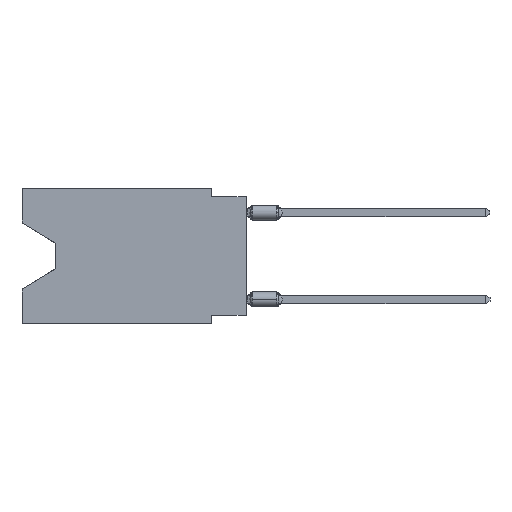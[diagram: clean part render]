
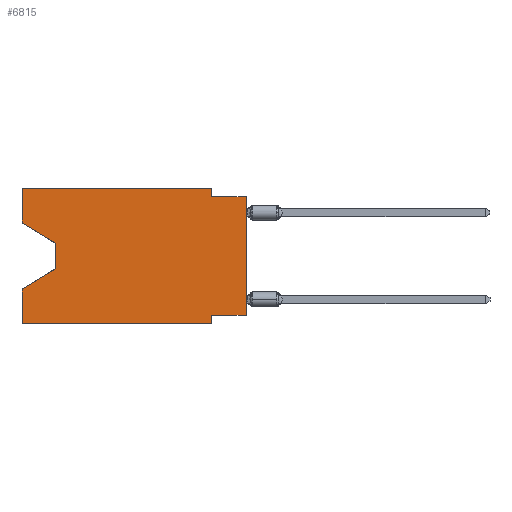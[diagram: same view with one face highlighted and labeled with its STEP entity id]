
A CAD part, left-side view. The second image highlights one B-rep face of the part: STEP entity #6815.
In plain terms, the highlighted planar face has unit normal (-1, 0, 0).
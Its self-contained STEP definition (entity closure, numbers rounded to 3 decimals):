
#292 = DIRECTION ( 'NONE',  ( 1., 0., 0. ) ) ;
#353 = VERTEX_POINT ( 'NONE', #10579 ) ;
#389 = EDGE_CURVE ( 'NONE', #13629, #1016, #3475, .T. ) ;
#968 = VECTOR ( 'NONE', #1400, 1000. ) ;
#1016 = VERTEX_POINT ( 'NONE', #14931 ) ;
#1067 = EDGE_CURVE ( 'NONE', #29259, #17591, #10344, .T. ) ;
#1400 = DIRECTION ( 'NONE',  ( 0., 0., 1. ) ) ;
#2330 = CARTESIAN_POINT ( 'NONE',  ( 0., 16.383, -9.906 ) ) ;
#2386 = CARTESIAN_POINT ( 'NONE',  ( 0., 0., -9.271 ) ) ;
#2411 = CARTESIAN_POINT ( 'NONE',  ( 0., 2.54, -9.906 ) ) ;
#3475 = LINE ( 'NONE', #3944, #26967 ) ;
#3944 = CARTESIAN_POINT ( 'NONE',  ( 0., 13.97, -4.013 ) ) ;
#4146 = VERTEX_POINT ( 'NONE', #13972 ) ;
#5473 = VECTOR ( 'NONE', #10708, 1000. ) ;
#5491 = LINE ( 'NONE', #27127, #30557 ) ;
#5962 = VECTOR ( 'NONE', #19684, 1000. ) ;
#6553 = DIRECTION ( 'NONE',  ( 0., -1., 0. ) ) ;
#6568 = CARTESIAN_POINT ( 'NONE',  ( 0., 0., -0.635 ) ) ;
#6754 = CARTESIAN_POINT ( 'NONE',  ( 0., 16.383, 0. ) ) ;
#6815 = ADVANCED_FACE ( 'NONE', ( #24852 ), #7393, .F. ) ;
#7220 = DIRECTION ( 'NONE',  ( 0., -1., 0. ) ) ;
#7393 = PLANE ( 'NONE',  #9376 ) ;
#7778 = CARTESIAN_POINT ( 'NONE',  ( 0., 16.383, -2.546 ) ) ;
#8778 = DIRECTION ( 'NONE',  ( 0., 1., 0. ) ) ;
#9224 = ORIENTED_EDGE ( 'NONE', *, *, #16966, .T. ) ;
#9267 = CARTESIAN_POINT ( 'NONE',  ( 0., 16.383, -9.906 ) ) ;
#9376 = AXIS2_PLACEMENT_3D ( 'NONE', #16717, #292, #19379 ) ;
#9583 = ORIENTED_EDGE ( 'NONE', *, *, #28936, .F. ) ;
#9595 = ORIENTED_EDGE ( 'NONE', *, *, #1067, .F. ) ;
#9764 = CARTESIAN_POINT ( 'NONE',  ( 0., 0., 0. ) ) ;
#10002 = DIRECTION ( 'NONE',  ( 0., -0.855, -0.519 ) ) ;
#10344 = LINE ( 'NONE', #22487, #17289 ) ;
#10445 = LINE ( 'NONE', #20059, #25078 ) ;
#10452 = LINE ( 'NONE', #7778, #21352 ) ;
#10579 = CARTESIAN_POINT ( 'NONE',  ( 0., 16.383, 0. ) ) ;
#10708 = DIRECTION ( 'NONE',  ( 0., 0., -1. ) ) ;
#12128 = VERTEX_POINT ( 'NONE', #2386 ) ;
#12500 = EDGE_CURVE ( 'NONE', #12128, #12822, #17470, .T. ) ;
#12691 = EDGE_CURVE ( 'NONE', #12128, #4146, #27576, .T. ) ;
#12791 = ORIENTED_EDGE ( 'NONE', *, *, #12691, .F. ) ;
#12822 = VERTEX_POINT ( 'NONE', #6568 ) ;
#12853 = CARTESIAN_POINT ( 'NONE',  ( 0., 16.383, -2.546 ) ) ;
#12899 = DIRECTION ( 'NONE',  ( 0., 0., 1. ) ) ;
#13097 = DIRECTION ( 'NONE',  ( 0., 0., -1. ) ) ;
#13191 = CARTESIAN_POINT ( 'NONE',  ( 0., 2.54, 0. ) ) ;
#13629 = VERTEX_POINT ( 'NONE', #16755 ) ;
#13839 = ORIENTED_EDGE ( 'NONE', *, *, #17500, .T. ) ;
#13948 = ORIENTED_EDGE ( 'NONE', *, *, #18404, .F. ) ;
#13972 = CARTESIAN_POINT ( 'NONE',  ( 0., 2.54, -9.271 ) ) ;
#14377 = EDGE_CURVE ( 'NONE', #1016, #14580, #25808, .T. ) ;
#14580 = VERTEX_POINT ( 'NONE', #27813 ) ;
#14851 = VECTOR ( 'NONE', #30859, 1000. ) ;
#14931 = CARTESIAN_POINT ( 'NONE',  ( 0., 13.97, -5.893 ) ) ;
#15387 = LINE ( 'NONE', #27873, #20533 ) ;
#15561 = VERTEX_POINT ( 'NONE', #9267 ) ;
#16714 = EDGE_CURVE ( 'NONE', #15561, #14580, #5491, .T. ) ;
#16717 = CARTESIAN_POINT ( 'NONE',  ( 0., 16.383, 0. ) ) ;
#16755 = CARTESIAN_POINT ( 'NONE',  ( 0., 13.97, -4.013 ) ) ;
#16966 = EDGE_CURVE ( 'NONE', #15561, #26094, #19047, .T. ) ;
#17289 = VECTOR ( 'NONE', #22645, 1000. ) ;
#17470 = LINE ( 'NONE', #9764, #5962 ) ;
#17500 = EDGE_CURVE ( 'NONE', #26839, #13629, #10452, .T. ) ;
#17532 = ORIENTED_EDGE ( 'NONE', *, *, #28760, .F. ) ;
#17591 = VERTEX_POINT ( 'NONE', #18341 ) ;
#17893 = ORIENTED_EDGE ( 'NONE', *, *, #389, .T. ) ;
#18341 = CARTESIAN_POINT ( 'NONE',  ( 0., 2.54, -0.635 ) ) ;
#18404 = EDGE_CURVE ( 'NONE', #17591, #12822, #15387, .T. ) ;
#19047 = LINE ( 'NONE', #2330, #24010 ) ;
#19379 = DIRECTION ( 'NONE',  ( 0., 0., -1. ) ) ;
#19684 = DIRECTION ( 'NONE',  ( 0., 0., 1. ) ) ;
#20052 = EDGE_CURVE ( 'NONE', #353, #29259, #10445, .T. ) ;
#20059 = CARTESIAN_POINT ( 'NONE',  ( 0., 16.383, 0. ) ) ;
#20137 = CARTESIAN_POINT ( 'NONE',  ( 0., 0., -9.271 ) ) ;
#20533 = VECTOR ( 'NONE', #6553, 1000. ) ;
#21215 = CARTESIAN_POINT ( 'NONE',  ( 0., 13.97, -5.893 ) ) ;
#21276 = LINE ( 'NONE', #6754, #968 ) ;
#21352 = VECTOR ( 'NONE', #10002, 1000. ) ;
#22487 = CARTESIAN_POINT ( 'NONE',  ( 0., 2.54, 0. ) ) ;
#22645 = DIRECTION ( 'NONE',  ( 0., 0., -1. ) ) ;
#22782 = ORIENTED_EDGE ( 'NONE', *, *, #16714, .F. ) ;
#24010 = VECTOR ( 'NONE', #7220, 1000. ) ;
#24620 = VECTOR ( 'NONE', #8778, 1000. ) ;
#24852 = FACE_OUTER_BOUND ( 'NONE', #27753, .T. ) ;
#24971 = DIRECTION ( 'NONE',  ( 0., -1., 0. ) ) ;
#25078 = VECTOR ( 'NONE', #24971, 1000. ) ;
#25808 = LINE ( 'NONE', #21215, #14851 ) ;
#25940 = CARTESIAN_POINT ( 'NONE',  ( 0., 2.54, -9.906 ) ) ;
#26094 = VERTEX_POINT ( 'NONE', #25940 ) ;
#26473 = ORIENTED_EDGE ( 'NONE', *, *, #20052, .F. ) ;
#26839 = VERTEX_POINT ( 'NONE', #12853 ) ;
#26967 = VECTOR ( 'NONE', #13097, 1000. ) ;
#27127 = CARTESIAN_POINT ( 'NONE',  ( 0., 16.383, 0. ) ) ;
#27576 = LINE ( 'NONE', #20137, #24620 ) ;
#27753 = EDGE_LOOP ( 'NONE', ( #13839, #17893, #29697, #22782, #9224, #17532, #12791, #30137, #13948, #9595, #26473, #9583 ) ) ;
#27813 = CARTESIAN_POINT ( 'NONE',  ( 0., 16.383, -7.36 ) ) ;
#27873 = CARTESIAN_POINT ( 'NONE',  ( 0., 0., -0.635 ) ) ;
#28760 = EDGE_CURVE ( 'NONE', #4146, #26094, #31147, .T. ) ;
#28936 = EDGE_CURVE ( 'NONE', #26839, #353, #21276, .T. ) ;
#29259 = VERTEX_POINT ( 'NONE', #13191 ) ;
#29697 = ORIENTED_EDGE ( 'NONE', *, *, #14377, .T. ) ;
#30137 = ORIENTED_EDGE ( 'NONE', *, *, #12500, .T. ) ;
#30557 = VECTOR ( 'NONE', #12899, 1000. ) ;
#30859 = DIRECTION ( 'NONE',  ( 0., 0.855, -0.519 ) ) ;
#31147 = LINE ( 'NONE', #2411, #5473 ) ;
